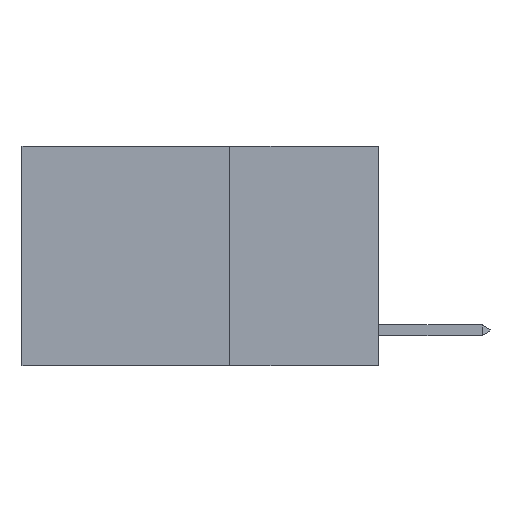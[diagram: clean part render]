
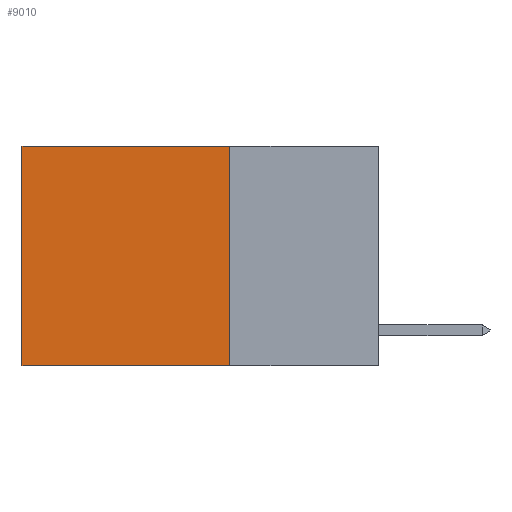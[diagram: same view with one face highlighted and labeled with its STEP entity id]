
A CAD part, left-side view. The second image highlights one B-rep face of the part: STEP entity #9010.
In plain terms, the highlighted planar face has unit normal (-1, 0, 0).
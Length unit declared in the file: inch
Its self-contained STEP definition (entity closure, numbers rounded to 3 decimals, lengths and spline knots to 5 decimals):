
#75 = CARTESIAN_POINT ( 'NONE',  ( 0.2625, 0.25, 0. ) ) ;
#253 = VERTEX_POINT ( 'NONE', #75 ) ;
#439 = ORIENTED_EDGE ( 'NONE', *, *, #1376, .F. ) ;
#1234 = VECTOR ( 'NONE', #1275, 39.37008 ) ;
#1275 = DIRECTION ( 'NONE',  ( 0., 1., 0. ) ) ;
#1376 = EDGE_CURVE ( 'NONE', #4706, #11575, #10416, .T. ) ;
#2753 = FACE_OUTER_BOUND ( 'NONE', #8407, .T. ) ;
#3223 = LINE ( 'NONE', #10866, #1234 ) ;
#3493 = ORIENTED_EDGE ( 'NONE', *, *, #8578, .T. ) ;
#3672 = CARTESIAN_POINT ( 'NONE',  ( 0.2625, 0.6, 0. ) ) ;
#4172 = EDGE_CURVE ( 'NONE', #253, #4706, #10514, .T. ) ;
#4552 = CARTESIAN_POINT ( 'NONE',  ( 0.2625, 0.25, -0.37 ) ) ;
#4706 = VERTEX_POINT ( 'NONE', #9978 ) ;
#4811 = LINE ( 'NONE', #5837, #9156 ) ;
#5537 = ORIENTED_EDGE ( 'NONE', *, *, #4172, .F. ) ;
#5837 = CARTESIAN_POINT ( 'NONE',  ( 0.2625, 0.6, 0. ) ) ;
#6385 = CARTESIAN_POINT ( 'NONE',  ( 0.2625, 0.6, -0.37 ) ) ;
#6620 = DIRECTION ( 'NONE',  ( 0., 0., -1. ) ) ;
#6721 = DIRECTION ( 'NONE',  ( 0., 0., -1. ) ) ;
#6774 = CARTESIAN_POINT ( 'NONE',  ( 0.2625, 0.25, 0. ) ) ;
#7525 = AXIS2_PLACEMENT_3D ( 'NONE', #6774, #9491, #10431 ) ;
#7539 = PLANE ( 'NONE',  #7525 ) ;
#7572 = CARTESIAN_POINT ( 'NONE',  ( 0.2625, 0.25, 0. ) ) ;
#7593 = DIRECTION ( 'NONE',  ( 0., 1., 0. ) ) ;
#8305 = EDGE_CURVE ( 'NONE', #253, #9718, #3223, .T. ) ;
#8321 = VECTOR ( 'NONE', #7593, 39.37008 ) ;
#8407 = EDGE_LOOP ( 'NONE', ( #3493, #439, #5537, #10860 ) ) ;
#8578 = EDGE_CURVE ( 'NONE', #9718, #11575, #4811, .T. ) ;
#9010 = ADVANCED_FACE ( 'NONE', ( #2753 ), #7539, .F. ) ;
#9156 = VECTOR ( 'NONE', #6721, 39.37008 ) ;
#9491 = DIRECTION ( 'NONE',  ( 1., 0., 0. ) ) ;
#9718 = VERTEX_POINT ( 'NONE', #3672 ) ;
#9978 = CARTESIAN_POINT ( 'NONE',  ( 0.2625, 0.25, -0.37 ) ) ;
#10416 = LINE ( 'NONE', #4552, #8321 ) ;
#10431 = DIRECTION ( 'NONE',  ( 0., 0., -1. ) ) ;
#10514 = LINE ( 'NONE', #7572, #11321 ) ;
#10860 = ORIENTED_EDGE ( 'NONE', *, *, #8305, .T. ) ;
#10866 = CARTESIAN_POINT ( 'NONE',  ( 0.2625, 0.25, 0. ) ) ;
#11321 = VECTOR ( 'NONE', #6620, 39.37008 ) ;
#11575 = VERTEX_POINT ( 'NONE', #6385 ) ;
